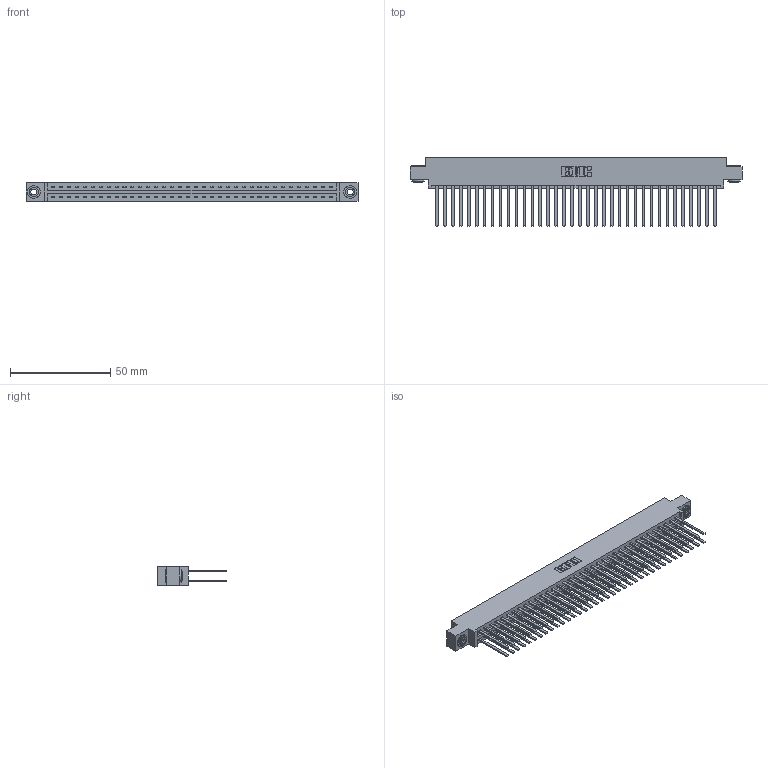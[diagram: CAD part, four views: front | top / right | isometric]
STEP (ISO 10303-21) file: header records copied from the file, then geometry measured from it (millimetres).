
FILE_DESCRIPTION (( 'STEP AP203' ), '1' );
FILE_NAME ('337-072-544-803.STEP', '2019-10-15T11:48:52', ( '' ), ( '' ), 'SwSTEP 2.0', 'SolidWorks 2016', '' );
FILE_SCHEMA (( 'CONFIG_CONTROL_DESIGN' ));
Length unit declared in the file: inch
Products named in the file (4): 337-072-544-803; 345-250-002_345-250-002-102; 337 Part_0.170 Offset - 0.156 Dia-TH; 345-292-001_345-293-144
Assembly tree (75 placements, depth 2):
  337-072-544-803
    337 Part_0.170 Offset - 0.156 Dia-TH
    345-292-001_345-293-144  x72
    345-250-002_345-250-002-102  x2
Bounding box: 165.66 x 34.3 x 9.4 mm (x, y, z)
Volume: 18289.8 mm3; surface area: 24247.7 mm2
Topology: 75 solids, 75 shells, 3612 faces, 10695 edges, 7030 vertices
Faces by surface type: plane 2532, cylinder 1072, cone 8
Entity records: 29286 total; most frequent: CARTESIAN_POINT 4913, ORIENTED_EDGE 4842, DIRECTION 4219, EDGE_CURVE 2421, LINE 2273, VECTOR 2273, VERTEX_POINT 1610, AXIS2_PLACEMENT_3D 973
